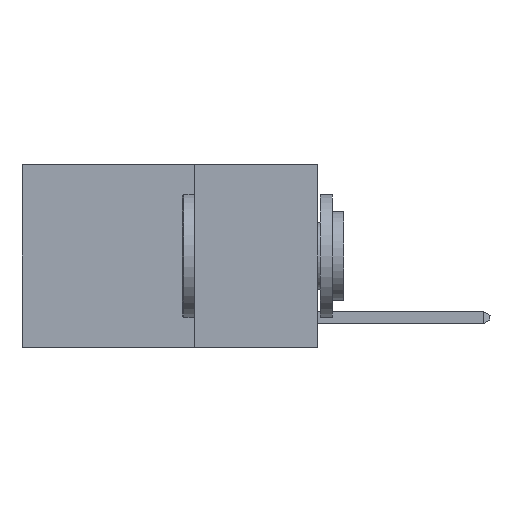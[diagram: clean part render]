
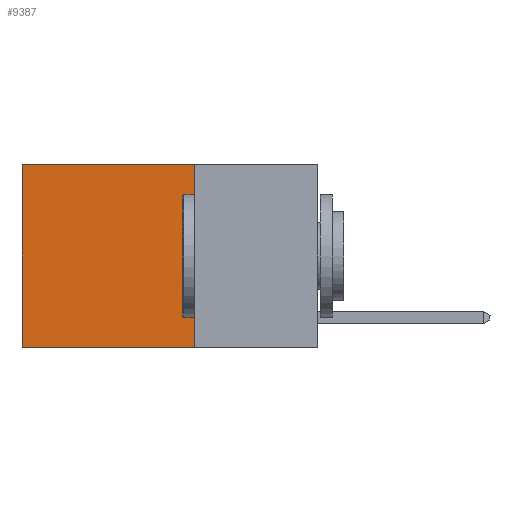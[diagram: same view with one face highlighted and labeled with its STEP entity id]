
A CAD part, left-side view. The second image highlights one B-rep face of the part: STEP entity #9387.
In plain terms, the highlighted planar face has unit normal (-1, 0, 0).
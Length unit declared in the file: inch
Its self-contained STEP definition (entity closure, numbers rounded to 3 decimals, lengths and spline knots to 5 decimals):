
#442 = VECTOR ( 'NONE', #21312, 39.37008 ) ;
#1174 = LINE ( 'NONE', #3375, #442 ) ;
#1649 = DIRECTION ( 'NONE',  ( 1., 0., 0. ) ) ;
#2069 = CARTESIAN_POINT ( 'NONE',  ( 0.2625, 0.6, 0. ) ) ;
#2907 = ORIENTED_EDGE ( 'NONE', *, *, #21060, .T. ) ;
#3134 = CARTESIAN_POINT ( 'NONE',  ( 0.2625, 0.25, 0. ) ) ;
#3375 = CARTESIAN_POINT ( 'NONE',  ( 0.2625, 0.25, -0.37 ) ) ;
#3857 = CARTESIAN_POINT ( 'NONE',  ( 0.2625, 0.25, 0. ) ) ;
#3881 = VERTEX_POINT ( 'NONE', #7220 ) ;
#3916 = DIRECTION ( 'NONE',  ( 0., 0., -1. ) ) ;
#5794 = VECTOR ( 'NONE', #18195, 39.37008 ) ;
#6568 = EDGE_CURVE ( 'NONE', #12824, #3881, #17156, .T. ) ;
#7220 = CARTESIAN_POINT ( 'NONE',  ( 0.2625, 0.25, -0.37 ) ) ;
#9220 = CARTESIAN_POINT ( 'NONE',  ( 0.2625, 0.25, 0. ) ) ;
#9387 = ADVANCED_FACE ( 'NONE', ( #16734 ), #23189, .F. ) ;
#10989 = VERTEX_POINT ( 'NONE', #22765 ) ;
#11009 = CARTESIAN_POINT ( 'NONE',  ( 0.2625, 0.6, 0. ) ) ;
#11546 = LINE ( 'NONE', #2069, #20418 ) ;
#11768 = LINE ( 'NONE', #3857, #5794 ) ;
#12499 = VERTEX_POINT ( 'NONE', #11009 ) ;
#12824 = VERTEX_POINT ( 'NONE', #3134 ) ;
#14406 = DIRECTION ( 'NONE',  ( 0., 0., -1. ) ) ;
#16170 = EDGE_LOOP ( 'NONE', ( #2907, #20506, #18191, #17186 ) ) ;
#16440 = AXIS2_PLACEMENT_3D ( 'NONE', #21424, #1649, #14406 ) ;
#16600 = VECTOR ( 'NONE', #21673, 39.37008 ) ;
#16734 = FACE_OUTER_BOUND ( 'NONE', #16170, .T. ) ;
#17156 = LINE ( 'NONE', #9220, #16600 ) ;
#17186 = ORIENTED_EDGE ( 'NONE', *, *, #22348, .T. ) ;
#18191 = ORIENTED_EDGE ( 'NONE', *, *, #6568, .F. ) ;
#18195 = DIRECTION ( 'NONE',  ( 0., 1., 0. ) ) ;
#20418 = VECTOR ( 'NONE', #3916, 39.37008 ) ;
#20506 = ORIENTED_EDGE ( 'NONE', *, *, #22183, .F. ) ;
#21060 = EDGE_CURVE ( 'NONE', #12499, #10989, #11546, .T. ) ;
#21312 = DIRECTION ( 'NONE',  ( 0., 1., 0. ) ) ;
#21424 = CARTESIAN_POINT ( 'NONE',  ( 0.2625, 0.25, 0. ) ) ;
#21673 = DIRECTION ( 'NONE',  ( 0., 0., -1. ) ) ;
#22183 = EDGE_CURVE ( 'NONE', #3881, #10989, #1174, .T. ) ;
#22348 = EDGE_CURVE ( 'NONE', #12824, #12499, #11768, .T. ) ;
#22765 = CARTESIAN_POINT ( 'NONE',  ( 0.2625, 0.6, -0.37 ) ) ;
#23189 = PLANE ( 'NONE',  #16440 ) ;
